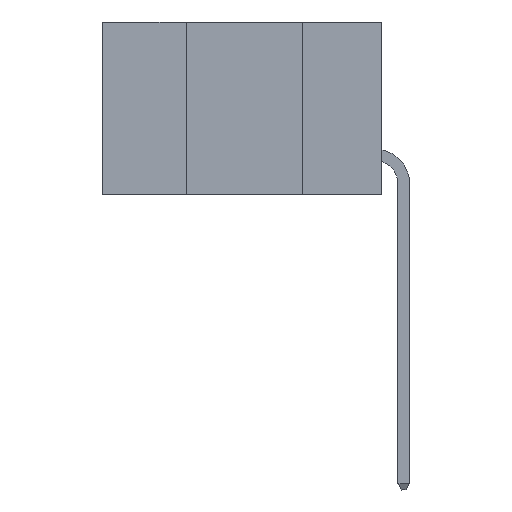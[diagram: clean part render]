
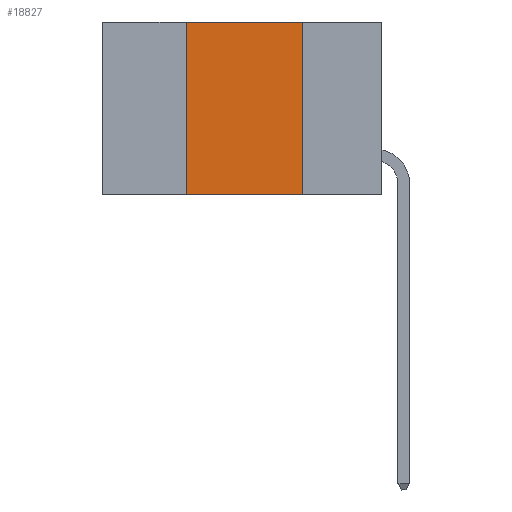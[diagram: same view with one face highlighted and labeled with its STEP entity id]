
A CAD part, left-side view. The second image highlights one B-rep face of the part: STEP entity #18827.
In plain terms, the highlighted planar face has unit normal (-1, 0, 0).
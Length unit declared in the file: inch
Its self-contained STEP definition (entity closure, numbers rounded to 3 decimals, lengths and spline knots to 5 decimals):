
#127 = ORIENTED_EDGE ( 'NONE', *, *, #4101, .F. ) ;
#803 = VECTOR ( 'NONE', #24222, 39.37008 ) ;
#1634 = VERTEX_POINT ( 'NONE', #8856 ) ;
#3224 = VERTEX_POINT ( 'NONE', #8604 ) ;
#3268 = VERTEX_POINT ( 'NONE', #10868 ) ;
#4101 = EDGE_CURVE ( 'NONE', #3224, #11685, #5597, .T. ) ;
#5597 = LINE ( 'NONE', #15353, #9852 ) ;
#5749 = CARTESIAN_POINT ( 'NONE',  ( 0., 0.6, 0. ) ) ;
#8104 = VECTOR ( 'NONE', #24400, 39.37008 ) ;
#8604 = CARTESIAN_POINT ( 'NONE',  ( 0., 0.17, 0. ) ) ;
#8856 = CARTESIAN_POINT ( 'NONE',  ( 0., 0.42, 0. ) ) ;
#9852 = VECTOR ( 'NONE', #15438, 39.37008 ) ;
#9950 = DIRECTION ( 'NONE',  ( 0., 0., -1. ) ) ;
#10594 = CARTESIAN_POINT ( 'NONE',  ( 0., 0.17, -0.37 ) ) ;
#10868 = CARTESIAN_POINT ( 'NONE',  ( 0., 0.42, -0.37 ) ) ;
#11040 = VECTOR ( 'NONE', #13299, 39.37008 ) ;
#11685 = VERTEX_POINT ( 'NONE', #10594 ) ;
#13299 = DIRECTION ( 'NONE',  ( 0., -1., 0. ) ) ;
#13611 = LINE ( 'NONE', #22378, #8104 ) ;
#13908 = EDGE_CURVE ( 'NONE', #1634, #3224, #21932, .T. ) ;
#14019 = ORIENTED_EDGE ( 'NONE', *, *, #13908, .F. ) ;
#14229 = EDGE_CURVE ( 'NONE', #3268, #11685, #13611, .T. ) ;
#14757 = FACE_OUTER_BOUND ( 'NONE', #22068, .T. ) ;
#15353 = CARTESIAN_POINT ( 'NONE',  ( 0., 0.17, 0. ) ) ;
#15438 = DIRECTION ( 'NONE',  ( 0., 0., -1. ) ) ;
#17611 = LINE ( 'NONE', #22221, #803 ) ;
#18827 = ADVANCED_FACE ( 'NONE', ( #14757 ), #20209, .F. ) ;
#19362 = EDGE_CURVE ( 'NONE', #3268, #1634, #17611, .T. ) ;
#19955 = ORIENTED_EDGE ( 'NONE', *, *, #19362, .F. ) ;
#20082 = AXIS2_PLACEMENT_3D ( 'NONE', #5749, #22247, #9950 ) ;
#20209 = PLANE ( 'NONE',  #20082 ) ;
#21932 = LINE ( 'NONE', #25475, #11040 ) ;
#22068 = EDGE_LOOP ( 'NONE', ( #127, #14019, #19955, #26688 ) ) ;
#22221 = CARTESIAN_POINT ( 'NONE',  ( 0., 0.42, 0. ) ) ;
#22247 = DIRECTION ( 'NONE',  ( 1., 0., 0. ) ) ;
#22378 = CARTESIAN_POINT ( 'NONE',  ( 0., 0.6, -0.37 ) ) ;
#24222 = DIRECTION ( 'NONE',  ( 0., 0., 1. ) ) ;
#24400 = DIRECTION ( 'NONE',  ( 0., -1., 0. ) ) ;
#25475 = CARTESIAN_POINT ( 'NONE',  ( 0., 0.6, 0. ) ) ;
#26688 = ORIENTED_EDGE ( 'NONE', *, *, #14229, .T. ) ;
